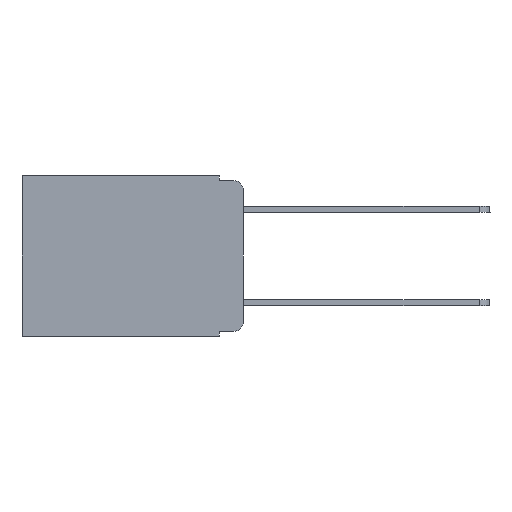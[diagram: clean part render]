
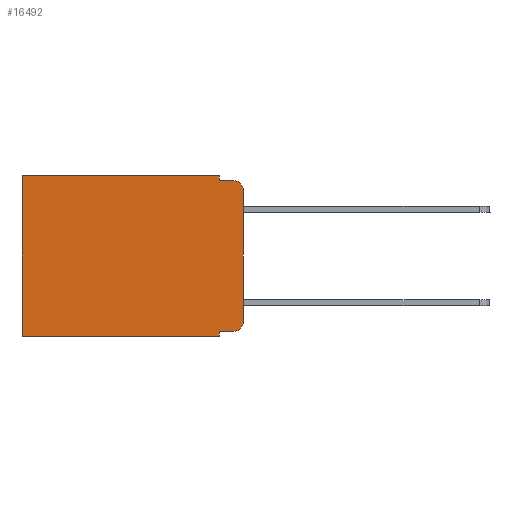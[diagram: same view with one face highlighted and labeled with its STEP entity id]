
A CAD part, left-side view. The second image highlights one B-rep face of the part: STEP entity #16492.
In plain terms, the highlighted planar face has unit normal (-1, 0, 0).
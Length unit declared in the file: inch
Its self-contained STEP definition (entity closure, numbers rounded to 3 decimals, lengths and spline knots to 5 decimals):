
#95 = ORIENTED_EDGE ( 'NONE', *, *, #16038, .T. ) ;
#1092 = DIRECTION ( 'NONE',  ( -1., 0., 0. ) ) ;
#1466 = VERTEX_POINT ( 'NONE', #16832 ) ;
#1698 = VERTEX_POINT ( 'NONE', #5528 ) ;
#1797 = ORIENTED_EDGE ( 'NONE', *, *, #6217, .F. ) ;
#2196 = CARTESIAN_POINT ( 'NONE',  ( 0.298, 0.051, -0.01 ) ) ;
#2449 = VERTEX_POINT ( 'NONE', #14153 ) ;
#2485 = DIRECTION ( 'NONE',  ( 0., 1., 0. ) ) ;
#3104 = CARTESIAN_POINT ( 'NONE',  ( 0.298, 0.051, 0. ) ) ;
#3383 = CARTESIAN_POINT ( 'NONE',  ( 0.298, 0., -0.343 ) ) ;
#3478 = PLANE ( 'NONE',  #16402 ) ;
#3856 = VECTOR ( 'NONE', #20106, 39.37008 ) ;
#4164 = DIRECTION ( 'NONE',  ( 0., 0., -1. ) ) ;
#4442 = EDGE_CURVE ( 'NONE', #22139, #21931, #21730, .T. ) ;
#4519 = CARTESIAN_POINT ( 'NONE',  ( 0.298, 0.051, 0. ) ) ;
#4672 = LINE ( 'NONE', #13236, #18344 ) ;
#4841 = VECTOR ( 'NONE', #19219, 39.37008 ) ;
#5528 = CARTESIAN_POINT ( 'NONE',  ( 0.298, 0.051, -0.333 ) ) ;
#5665 = LINE ( 'NONE', #12742, #22222 ) ;
#5782 = DIRECTION ( 'NONE',  ( 0., -1., 0. ) ) ;
#5867 = DIRECTION ( 'NONE',  ( 0., 0., -1. ) ) ;
#5985 = DIRECTION ( 'NONE',  ( 1., 0., 0. ) ) ;
#6028 = VERTEX_POINT ( 'NONE', #8148 ) ;
#6138 = AXIS2_PLACEMENT_3D ( 'NONE', #16682, #1092, #4164 ) ;
#6152 = ORIENTED_EDGE ( 'NONE', *, *, #10761, .T. ) ;
#6217 = EDGE_CURVE ( 'NONE', #6028, #14363, #21035, .T. ) ;
#6222 = LINE ( 'NONE', #13176, #3856 ) ;
#6278 = VECTOR ( 'NONE', #2485, 39.37008 ) ;
#6769 = ORIENTED_EDGE ( 'NONE', *, *, #9313, .F. ) ;
#6805 = VECTOR ( 'NONE', #9772, 39.37008 ) ;
#7145 = EDGE_CURVE ( 'NONE', #21931, #14363, #4672, .T. ) ;
#7926 = CARTESIAN_POINT ( 'NONE',  ( 0.298, 0., 0. ) ) ;
#8148 = CARTESIAN_POINT ( 'NONE',  ( 0.298, 0.051, -0.343 ) ) ;
#8730 = FACE_OUTER_BOUND ( 'NONE', #16259, .T. ) ;
#9313 = EDGE_CURVE ( 'NONE', #22139, #12118, #19892, .T. ) ;
#9688 = ORIENTED_EDGE ( 'NONE', *, *, #7145, .T. ) ;
#9772 = DIRECTION ( 'NONE',  ( 0., 0., -1. ) ) ;
#10194 = CARTESIAN_POINT ( 'NONE',  ( 0.298, 0.02, -0.03 ) ) ;
#10241 = ORIENTED_EDGE ( 'NONE', *, *, #4442, .T. ) ;
#10458 = CARTESIAN_POINT ( 'NONE',  ( 0.298, 0., 0. ) ) ;
#10761 = EDGE_CURVE ( 'NONE', #2449, #19751, #22096, .T. ) ;
#11099 = LINE ( 'NONE', #11540, #18600 ) ;
#11250 = CIRCLE ( 'NONE', #6138, 0.02 ) ;
#11540 = CARTESIAN_POINT ( 'NONE',  ( 0.298, 0.051, 0. ) ) ;
#11681 = ORIENTED_EDGE ( 'NONE', *, *, #11880, .F. ) ;
#11880 = EDGE_CURVE ( 'NONE', #2449, #13734, #21920, .T. ) ;
#11898 = DIRECTION ( 'NONE',  ( 0., 0., -1. ) ) ;
#11931 = EDGE_CURVE ( 'NONE', #1466, #13734, #11250, .T. ) ;
#12118 = VERTEX_POINT ( 'NONE', #2196 ) ;
#12742 = CARTESIAN_POINT ( 'NONE',  ( 0.298, 0.051, -0.333 ) ) ;
#13089 = CARTESIAN_POINT ( 'NONE',  ( 0.298, 0., 0. ) ) ;
#13176 = CARTESIAN_POINT ( 'NONE',  ( 0.298, 0.051, -0.01 ) ) ;
#13236 = CARTESIAN_POINT ( 'NONE',  ( 0.298, 0.473, 0. ) ) ;
#13303 = ORIENTED_EDGE ( 'NONE', *, *, #11931, .T. ) ;
#13734 = VERTEX_POINT ( 'NONE', #14965 ) ;
#13761 = VECTOR ( 'NONE', #21578, 39.37008 ) ;
#14153 = CARTESIAN_POINT ( 'NONE',  ( 0.298, 0., -0.03 ) ) ;
#14363 = VERTEX_POINT ( 'NONE', #22077 ) ;
#14965 = CARTESIAN_POINT ( 'NONE',  ( 0.298, 0., -0.313 ) ) ;
#15112 = EDGE_CURVE ( 'NONE', #1698, #6028, #11099, .T. ) ;
#15549 = ORIENTED_EDGE ( 'NONE', *, *, #15112, .F. ) ;
#16038 = EDGE_CURVE ( 'NONE', #1698, #1466, #5665, .T. ) ;
#16259 = EDGE_LOOP ( 'NONE', ( #11681, #6152, #19098, #6769, #10241, #9688, #1797, #15549, #95, #13303 ) ) ;
#16402 = AXIS2_PLACEMENT_3D ( 'NONE', #10458, #5985, #5867 ) ;
#16492 = ADVANCED_FACE ( 'NONE', ( #8730 ), #3478, .F. ) ;
#16529 = DIRECTION ( 'NONE',  ( 0., 0., -1. ) ) ;
#16682 = CARTESIAN_POINT ( 'NONE',  ( 0.298, 0.02, -0.313 ) ) ;
#16832 = CARTESIAN_POINT ( 'NONE',  ( 0.298, 0.02, -0.333 ) ) ;
#17372 = CARTESIAN_POINT ( 'NONE',  ( 0.298, 0.473, 0. ) ) ;
#17744 = AXIS2_PLACEMENT_3D ( 'NONE', #10194, #18952, #11898 ) ;
#18344 = VECTOR ( 'NONE', #16529, 39.37008 ) ;
#18469 = DIRECTION ( 'NONE',  ( 0., 0., -1. ) ) ;
#18600 = VECTOR ( 'NONE', #18469, 39.37008 ) ;
#18952 = DIRECTION ( 'NONE',  ( -1., 0., 0. ) ) ;
#19098 = ORIENTED_EDGE ( 'NONE', *, *, #20433, .F. ) ;
#19219 = DIRECTION ( 'NONE',  ( 0., 1., 0. ) ) ;
#19573 = CARTESIAN_POINT ( 'NONE',  ( 0.298, 0.02, -0.01 ) ) ;
#19751 = VERTEX_POINT ( 'NONE', #19573 ) ;
#19892 = LINE ( 'NONE', #4519, #6805 ) ;
#20106 = DIRECTION ( 'NONE',  ( 0., -1., 0. ) ) ;
#20433 = EDGE_CURVE ( 'NONE', #12118, #19751, #6222, .T. ) ;
#21035 = LINE ( 'NONE', #3383, #4841 ) ;
#21578 = DIRECTION ( 'NONE',  ( 0., 0., -1. ) ) ;
#21730 = LINE ( 'NONE', #13089, #6278 ) ;
#21920 = LINE ( 'NONE', #7926, #13761 ) ;
#21931 = VERTEX_POINT ( 'NONE', #17372 ) ;
#22077 = CARTESIAN_POINT ( 'NONE',  ( 0.298, 0.473, -0.343 ) ) ;
#22096 = CIRCLE ( 'NONE', #17744, 0.02 ) ;
#22139 = VERTEX_POINT ( 'NONE', #3104 ) ;
#22222 = VECTOR ( 'NONE', #5782, 39.37008 ) ;
